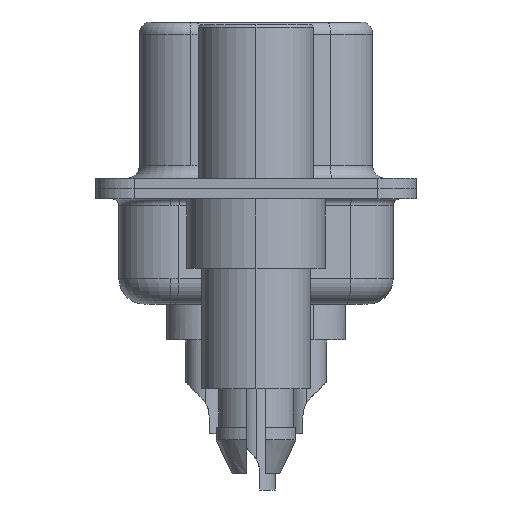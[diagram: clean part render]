
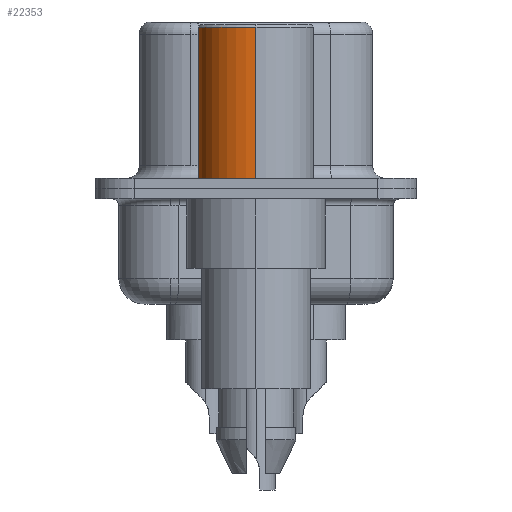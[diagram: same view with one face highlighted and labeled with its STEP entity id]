
A CAD part, left-side view. The second image highlights one B-rep face of the part: STEP entity #22353.
In plain terms, the highlighted cylindrical face has radius 2.25 mm (diameter 4.5 mm), a partial arc.
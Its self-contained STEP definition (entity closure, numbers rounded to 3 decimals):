
#1068 = CARTESIAN_POINT ( 'NONE',  ( 2.25, 0., 6.3 ) ) ;
#1215 = EDGE_LOOP ( 'NONE', ( #24300, #19381, #19707, #26886 ) ) ;
#2466 = CIRCLE ( 'NONE', #13860, 2.25 ) ;
#4087 = VERTEX_POINT ( 'NONE', #1068 ) ;
#4165 = DIRECTION ( 'NONE',  ( 0., 0., 1. ) ) ;
#4839 = CARTESIAN_POINT ( 'NONE',  ( -2.25, 0., 0.581 ) ) ;
#6685 = VECTOR ( 'NONE', #9166, 1000. ) ;
#7185 = VERTEX_POINT ( 'NONE', #7259 ) ;
#7259 = CARTESIAN_POINT ( 'NONE',  ( -2.25, 0., 6.3 ) ) ;
#7570 = AXIS2_PLACEMENT_3D ( 'NONE', #17110, #4165, #19165 ) ;
#9166 = DIRECTION ( 'NONE',  ( 0., 0., 1. ) ) ;
#10144 = CIRCLE ( 'NONE', #7570, 2.25 ) ;
#10307 = LINE ( 'NONE', #4839, #26280 ) ;
#11530 = DIRECTION ( 'NONE',  ( 1., 0., 0. ) ) ;
#11684 = VERTEX_POINT ( 'NONE', #20262 ) ;
#11705 = FACE_OUTER_BOUND ( 'NONE', #1215, .T. ) ;
#12138 = AXIS2_PLACEMENT_3D ( 'NONE', #24000, #13589, #11530 ) ;
#12376 = DIRECTION ( 'NONE',  ( 0., 0., 1. ) ) ;
#12437 = LINE ( 'NONE', #15421, #6685 ) ;
#13540 = VERTEX_POINT ( 'NONE', #16390 ) ;
#13589 = DIRECTION ( 'NONE',  ( 0., 0., 1. ) ) ;
#13860 = AXIS2_PLACEMENT_3D ( 'NONE', #24807, #12376, #26892 ) ;
#15421 = CARTESIAN_POINT ( 'NONE',  ( 2.25, 0., 0.581 ) ) ;
#16390 = CARTESIAN_POINT ( 'NONE',  ( 2.25, 0., 0.4 ) ) ;
#17110 = CARTESIAN_POINT ( 'NONE',  ( 0., 0., 0.4 ) ) ;
#19115 = EDGE_CURVE ( 'NONE', #4087, #7185, #2466, .T. ) ;
#19165 = DIRECTION ( 'NONE',  ( 1., 0., 0. ) ) ;
#19304 = EDGE_CURVE ( 'NONE', #13540, #11684, #10144, .T. ) ;
#19381 = ORIENTED_EDGE ( 'NONE', *, *, #23477, .T. ) ;
#19707 = ORIENTED_EDGE ( 'NONE', *, *, #19115, .F. ) ;
#20262 = CARTESIAN_POINT ( 'NONE',  ( -2.25, 0., 0.4 ) ) ;
#22353 = ADVANCED_FACE ( 'NONE', ( #11705 ), #27622, .T. ) ;
#23477 = EDGE_CURVE ( 'NONE', #11684, #7185, #10307, .T. ) ;
#24000 = CARTESIAN_POINT ( 'NONE',  ( 0., 0., 0.581 ) ) ;
#24300 = ORIENTED_EDGE ( 'NONE', *, *, #19304, .T. ) ;
#24807 = CARTESIAN_POINT ( 'NONE',  ( 0., 0., 6.3 ) ) ;
#26102 = DIRECTION ( 'NONE',  ( 0., 0., 1. ) ) ;
#26280 = VECTOR ( 'NONE', #26102, 1000. ) ;
#26886 = ORIENTED_EDGE ( 'NONE', *, *, #27647, .F. ) ;
#26892 = DIRECTION ( 'NONE',  ( 1., 0., 0. ) ) ;
#27622 = CYLINDRICAL_SURFACE ( 'NONE', #12138, 2.25 ) ;
#27647 = EDGE_CURVE ( 'NONE', #13540, #4087, #12437, .T. ) ;
